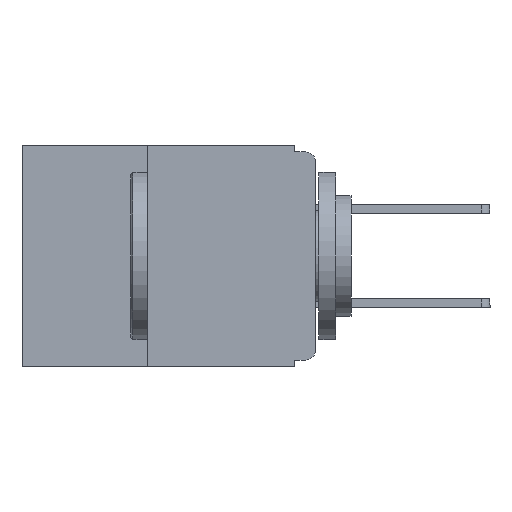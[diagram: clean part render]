
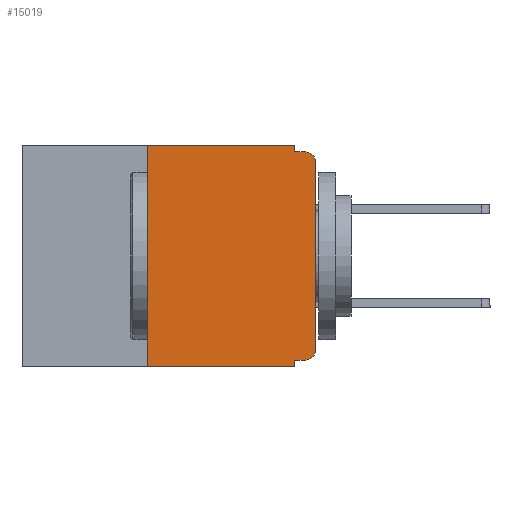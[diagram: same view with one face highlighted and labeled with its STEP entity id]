
A CAD part, left-side view. The second image highlights one B-rep face of the part: STEP entity #15019.
In plain terms, the highlighted planar face has unit normal (-1, 0, 0).
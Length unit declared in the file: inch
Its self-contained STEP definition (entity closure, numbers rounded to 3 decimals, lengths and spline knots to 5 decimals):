
#23 = ORIENTED_EDGE ( 'NONE', *, *, #6758, .T. ) ;
#75 = VECTOR ( 'NONE', #3852, 39.37008 ) ;
#429 = VECTOR ( 'NONE', #18811, 39.37008 ) ;
#436 = ORIENTED_EDGE ( 'NONE', *, *, #8672, .F. ) ;
#825 = ORIENTED_EDGE ( 'NONE', *, *, #15975, .T. ) ;
#1406 = CARTESIAN_POINT ( 'NONE',  ( 0., 0.031, -0.33 ) ) ;
#1474 = ORIENTED_EDGE ( 'NONE', *, *, #1729, .F. ) ;
#1599 = CARTESIAN_POINT ( 'NONE',  ( 0., 0., -0.01 ) ) ;
#1602 = LINE ( 'NONE', #18924, #429 ) ;
#1729 = EDGE_CURVE ( 'NONE', #4279, #7240, #1602, .T. ) ;
#1922 = CARTESIAN_POINT ( 'NONE',  ( 0., 0.031, 0. ) ) ;
#2001 = VECTOR ( 'NONE', #6186, 39.37008 ) ;
#2029 = DIRECTION ( 'NONE',  ( 0., 0., 1. ) ) ;
#2037 = ORIENTED_EDGE ( 'NONE', *, *, #10949, .F. ) ;
#2054 = EDGE_LOOP ( 'NONE', ( #23, #17284, #436, #6983, #12301, #15566, #825, #1474, #2037, #4110 ) ) ;
#2164 = EDGE_CURVE ( 'NONE', #12804, #4305, #7152, .T. ) ;
#2331 = CARTESIAN_POINT ( 'NONE',  ( 0., 0., 0. ) ) ;
#2559 = VERTEX_POINT ( 'NONE', #15505 ) ;
#3211 = CARTESIAN_POINT ( 'NONE',  ( 0., 0.25, -0.33 ) ) ;
#3474 = VERTEX_POINT ( 'NONE', #19156 ) ;
#3482 = VERTEX_POINT ( 'NONE', #4623 ) ;
#3852 = DIRECTION ( 'NONE',  ( 0., 0., -1. ) ) ;
#4085 = CIRCLE ( 'NONE', #5511, 0.015 ) ;
#4110 = ORIENTED_EDGE ( 'NONE', *, *, #20693, .T. ) ;
#4279 = VERTEX_POINT ( 'NONE', #12131 ) ;
#4305 = VERTEX_POINT ( 'NONE', #11441 ) ;
#4623 = CARTESIAN_POINT ( 'NONE',  ( 0., 0.015, -0.01 ) ) ;
#4940 = CARTESIAN_POINT ( 'NONE',  ( 0., 0., -0.305 ) ) ;
#5511 = AXIS2_PLACEMENT_3D ( 'NONE', #9964, #21864, #11756 ) ;
#6186 = DIRECTION ( 'NONE',  ( 0., 1., 0. ) ) ;
#6269 = CARTESIAN_POINT ( 'NONE',  ( 0., 0., -0.32 ) ) ;
#6758 = EDGE_CURVE ( 'NONE', #8642, #10207, #9478, .T. ) ;
#6983 = ORIENTED_EDGE ( 'NONE', *, *, #14080, .F. ) ;
#6984 = LINE ( 'NONE', #7825, #16287 ) ;
#7152 = LINE ( 'NONE', #7524, #20326 ) ;
#7240 = VERTEX_POINT ( 'NONE', #1406 ) ;
#7521 = VERTEX_POINT ( 'NONE', #18666 ) ;
#7524 = CARTESIAN_POINT ( 'NONE',  ( 0., 0.25, -0.33 ) ) ;
#7731 = DIRECTION ( 'NONE',  ( 0., 0., 1. ) ) ;
#7825 = CARTESIAN_POINT ( 'NONE',  ( 0., 0.437, 0. ) ) ;
#8642 = VERTEX_POINT ( 'NONE', #4940 ) ;
#8672 = EDGE_CURVE ( 'NONE', #7521, #3482, #12937, .T. ) ;
#8775 = FACE_OUTER_BOUND ( 'NONE', #2054, .T. ) ;
#9437 = DIRECTION ( 'NONE',  ( 0., -1., 0. ) ) ;
#9478 = LINE ( 'NONE', #2331, #17052 ) ;
#9704 = DIRECTION ( 'NONE',  ( 0., -1., 0. ) ) ;
#9964 = CARTESIAN_POINT ( 'NONE',  ( 0., 0.015, -0.305 ) ) ;
#10207 = VERTEX_POINT ( 'NONE', #11507 ) ;
#10215 = CARTESIAN_POINT ( 'NONE',  ( 0., 0.437, 0. ) ) ;
#10630 = DIRECTION ( 'NONE',  ( 0., 0., -1. ) ) ;
#10658 = DIRECTION ( 'NONE',  ( -1., 0., 0. ) ) ;
#10700 = CARTESIAN_POINT ( 'NONE',  ( 0., 0.015, -0.025 ) ) ;
#10843 = EDGE_CURVE ( 'NONE', #10207, #3482, #17901, .T. ) ;
#10949 = EDGE_CURVE ( 'NONE', #2559, #4279, #20689, .T. ) ;
#11441 = CARTESIAN_POINT ( 'NONE',  ( 0., 0.25, 0. ) ) ;
#11507 = CARTESIAN_POINT ( 'NONE',  ( 0., 0., -0.025 ) ) ;
#11756 = DIRECTION ( 'NONE',  ( 0., 0., -1. ) ) ;
#12015 = DIRECTION ( 'NONE',  ( 0., 0., -1. ) ) ;
#12131 = CARTESIAN_POINT ( 'NONE',  ( 0., 0.031, -0.32 ) ) ;
#12301 = ORIENTED_EDGE ( 'NONE', *, *, #20536, .F. ) ;
#12804 = VERTEX_POINT ( 'NONE', #3211 ) ;
#12937 = LINE ( 'NONE', #1599, #21903 ) ;
#14080 = EDGE_CURVE ( 'NONE', #3474, #7521, #14542, .T. ) ;
#14476 = AXIS2_PLACEMENT_3D ( 'NONE', #10700, #10658, #10630 ) ;
#14542 = LINE ( 'NONE', #1922, #75 ) ;
#14968 = AXIS2_PLACEMENT_3D ( 'NONE', #10215, #22116, #12015 ) ;
#15019 = ADVANCED_FACE ( 'NONE', ( #8775 ), #17023, .F. ) ;
#15505 = CARTESIAN_POINT ( 'NONE',  ( 0., 0.015, -0.32 ) ) ;
#15566 = ORIENTED_EDGE ( 'NONE', *, *, #2164, .F. ) ;
#15975 = EDGE_CURVE ( 'NONE', #12804, #7240, #21266, .T. ) ;
#16287 = VECTOR ( 'NONE', #19836, 39.37008 ) ;
#16338 = CARTESIAN_POINT ( 'NONE',  ( 0., 0.437, -0.33 ) ) ;
#17023 = PLANE ( 'NONE',  #14968 ) ;
#17052 = VECTOR ( 'NONE', #2029, 39.37008 ) ;
#17284 = ORIENTED_EDGE ( 'NONE', *, *, #10843, .T. ) ;
#17901 = CIRCLE ( 'NONE', #14476, 0.015 ) ;
#18666 = CARTESIAN_POINT ( 'NONE',  ( 0., 0.031, -0.01 ) ) ;
#18811 = DIRECTION ( 'NONE',  ( 0., 0., -1. ) ) ;
#18924 = CARTESIAN_POINT ( 'NONE',  ( 0., 0.031, -0.33 ) ) ;
#19156 = CARTESIAN_POINT ( 'NONE',  ( 0., 0.031, 0. ) ) ;
#19836 = DIRECTION ( 'NONE',  ( 0., -1., 0. ) ) ;
#20326 = VECTOR ( 'NONE', #7731, 39.37008 ) ;
#20536 = EDGE_CURVE ( 'NONE', #4305, #3474, #6984, .T. ) ;
#20689 = LINE ( 'NONE', #6269, #2001 ) ;
#20693 = EDGE_CURVE ( 'NONE', #2559, #8642, #4085, .T. ) ;
#20746 = VECTOR ( 'NONE', #9437, 39.37008 ) ;
#21266 = LINE ( 'NONE', #16338, #20746 ) ;
#21864 = DIRECTION ( 'NONE',  ( -1., 0., 0. ) ) ;
#21903 = VECTOR ( 'NONE', #9704, 39.37008 ) ;
#22116 = DIRECTION ( 'NONE',  ( 1., 0., 0. ) ) ;
